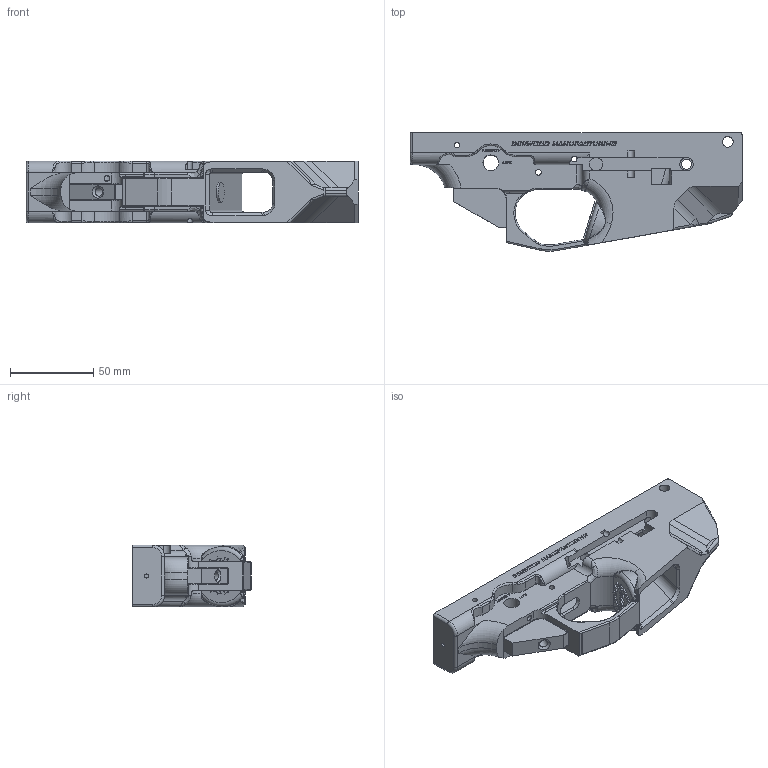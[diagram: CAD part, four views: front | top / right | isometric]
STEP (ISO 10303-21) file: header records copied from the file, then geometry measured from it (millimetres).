
FILE_DESCRIPTION(/* description */ ('','CAx-IF Rec.Pracs.---Representation and Presentation of Product Manufacturing Information (PMI)---3.8---2014-02-18'),/* implementation_level */ '2;1');
FILE_NAME(/* name */ 'WTF-9H Patriot Lower fix.stp',/* time_stamp */ '2020-05-13T13:04:48-07:00',/* author */ ('Uber Lobster'),/* organization */ (''),/* preprocessor_version */ 'ST-DEVELOPER v16.13',/* originating_system */ 'Autodesk Inventor 2018',/* authorisation */ '');
FILE_SCHEMA (('AP242_MANAGED_MODEL_BASED_3D_ENGINEERING_MIM_LF { 1 0 10303 442 1 1 4 }'));
Products named in the file (1): WTF-9H Patriot Lower
Bounding box: 199.47 x 71.26 x 37.13 mm (x, y, z)
Volume: 192492.5 mm3; surface area: 55271 mm2
Topology: 2 solids, 2 shells, 1671 faces, 4503 edges, 2958 vertices
Faces by surface type: plane 1220, bspline 262, cylinder 142, torus 43, sphere 2, cone 2
Full cylindrical faces by diameter (mm): 2.5 x1, 3 x1, 3.175 x3, 3.469 x4, 5.105 x1, 6 x1, 6.4 x2, 8 x1, 9.525 x2, 12 x1, 16.2 x1
Entity records: 64247 total; most frequent: CARTESIAN_POINT 22161, ORIENTED_EDGE 8924, DIRECTION 7134, EDGE_CURVE 4462, LINE 3524, VECTOR 3524, VERTEX_POINT 2948, EDGE_LOOP 1858
